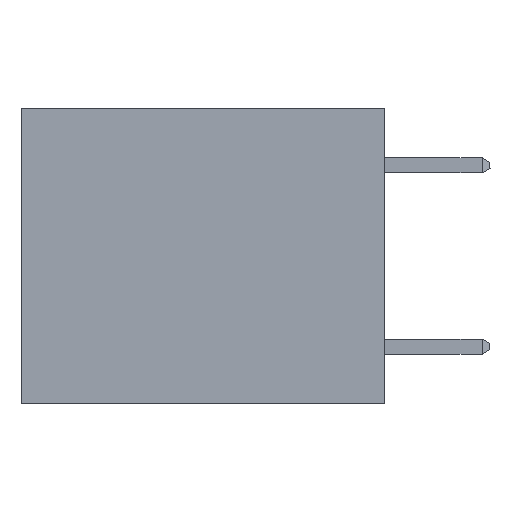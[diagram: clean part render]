
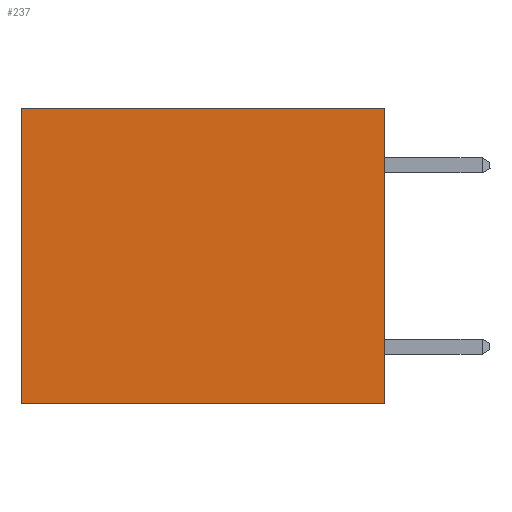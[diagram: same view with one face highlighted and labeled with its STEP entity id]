
A CAD part, left-side view. The second image highlights one B-rep face of the part: STEP entity #237.
In plain terms, the highlighted planar face has unit normal (-1, 0, 0).
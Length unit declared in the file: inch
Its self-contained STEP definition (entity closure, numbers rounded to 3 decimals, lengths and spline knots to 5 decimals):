
#237 = ADVANCED_FACE ( 'NONE', ( #18221 ), #11143, .F. ) ;
#397 = EDGE_CURVE ( 'NONE', #13731, #19852, #3045, .T. ) ;
#1141 = DIRECTION ( 'NONE',  ( 1., 0., 0. ) ) ;
#1487 = DIRECTION ( 'NONE',  ( 0., 0., -1. ) ) ;
#1818 = VECTOR ( 'NONE', #10699, 39.37008 ) ;
#2574 = ORIENTED_EDGE ( 'NONE', *, *, #11878, .T. ) ;
#3045 = LINE ( 'NONE', #14701, #15395 ) ;
#3651 = VECTOR ( 'NONE', #22042, 39.37008 ) ;
#3839 = CARTESIAN_POINT ( 'NONE',  ( 0.3165, 0.6, -0.49 ) ) ;
#4575 = EDGE_CURVE ( 'NONE', #21164, #18411, #7211, .T. ) ;
#4996 = CARTESIAN_POINT ( 'NONE',  ( 0.3165, 0., 0. ) ) ;
#6075 = EDGE_CURVE ( 'NONE', #21164, #13731, #20837, .T. ) ;
#7211 = LINE ( 'NONE', #13022, #1818 ) ;
#7835 = CARTESIAN_POINT ( 'NONE',  ( 0.3165, 0.6, 0. ) ) ;
#8547 = DIRECTION ( 'NONE',  ( 0., 1., 0. ) ) ;
#10699 = DIRECTION ( 'NONE',  ( 0., 1., 0. ) ) ;
#11143 = PLANE ( 'NONE',  #19678 ) ;
#11300 = VECTOR ( 'NONE', #22560, 39.37008 ) ;
#11878 = EDGE_CURVE ( 'NONE', #18411, #19852, #15998, .T. ) ;
#13022 = CARTESIAN_POINT ( 'NONE',  ( 0.3165, 0., 0. ) ) ;
#13731 = VERTEX_POINT ( 'NONE', #20656 ) ;
#14701 = CARTESIAN_POINT ( 'NONE',  ( 0.3165, 0., -0.49 ) ) ;
#15395 = VECTOR ( 'NONE', #8547, 39.37008 ) ;
#15998 = LINE ( 'NONE', #3839, #3651 ) ;
#18221 = FACE_OUTER_BOUND ( 'NONE', #22408, .T. ) ;
#18411 = VERTEX_POINT ( 'NONE', #7835 ) ;
#19292 = CARTESIAN_POINT ( 'NONE',  ( 0.3165, 0., -0.49 ) ) ;
#19678 = AXIS2_PLACEMENT_3D ( 'NONE', #19292, #1141, #1487 ) ;
#19852 = VERTEX_POINT ( 'NONE', #22387 ) ;
#20656 = CARTESIAN_POINT ( 'NONE',  ( 0.3165, 0., -0.49 ) ) ;
#20837 = LINE ( 'NONE', #21953, #11300 ) ;
#21164 = VERTEX_POINT ( 'NONE', #4996 ) ;
#21953 = CARTESIAN_POINT ( 'NONE',  ( 0.3165, 0., -0.49 ) ) ;
#22042 = DIRECTION ( 'NONE',  ( 0., 0., -1. ) ) ;
#22387 = CARTESIAN_POINT ( 'NONE',  ( 0.3165, 0.6, -0.49 ) ) ;
#22408 = EDGE_LOOP ( 'NONE', ( #2574, #25914, #24681, #23666 ) ) ;
#22560 = DIRECTION ( 'NONE',  ( 0., 0., -1. ) ) ;
#23666 = ORIENTED_EDGE ( 'NONE', *, *, #4575, .T. ) ;
#24681 = ORIENTED_EDGE ( 'NONE', *, *, #6075, .F. ) ;
#25914 = ORIENTED_EDGE ( 'NONE', *, *, #397, .F. ) ;
